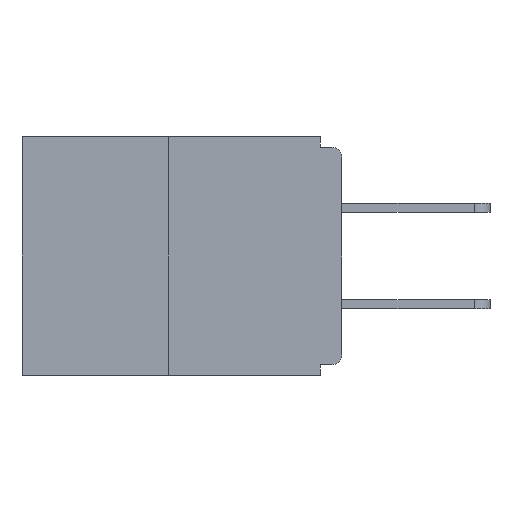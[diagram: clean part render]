
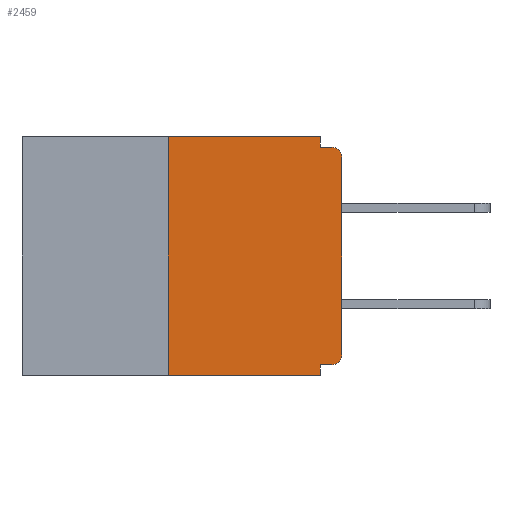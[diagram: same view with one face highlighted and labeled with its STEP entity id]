
A CAD part, left-side view. The second image highlights one B-rep face of the part: STEP entity #2459.
In plain terms, the highlighted planar face has unit normal (-1, 0, 0).
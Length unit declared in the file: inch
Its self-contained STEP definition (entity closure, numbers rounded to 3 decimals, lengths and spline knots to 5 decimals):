
#286 = DIRECTION ( 'NONE',  ( 0., 1., 0. ) ) ;
#424 = ORIENTED_EDGE ( 'NONE', *, *, #5537, .F. ) ;
#671 = CARTESIAN_POINT ( 'NONE',  ( 0., 0.015, -0.015 ) ) ;
#722 = FACE_OUTER_BOUND ( 'NONE', #28227, .T. ) ;
#727 = VECTOR ( 'NONE', #286, 39.37008 ) ;
#1129 = CARTESIAN_POINT ( 'NONE',  ( 0., 0., -0.015 ) ) ;
#1181 = ORIENTED_EDGE ( 'NONE', *, *, #14815, .F. ) ;
#1460 = EDGE_CURVE ( 'NONE', #25315, #20124, #7618, .T. ) ;
#1823 = VECTOR ( 'NONE', #16786, 39.37008 ) ;
#1989 = CARTESIAN_POINT ( 'NONE',  ( 0., 0.031, -0.343 ) ) ;
#2459 = ADVANCED_FACE ( 'NONE', ( #722 ), #16850, .F. ) ;
#2761 = VERTEX_POINT ( 'NONE', #17500 ) ;
#2852 = AXIS2_PLACEMENT_3D ( 'NONE', #22401, #15480, #24294 ) ;
#2941 = EDGE_CURVE ( 'NONE', #11455, #20124, #27939, .T. ) ;
#3742 = LINE ( 'NONE', #1129, #14697 ) ;
#5002 = VERTEX_POINT ( 'NONE', #21702 ) ;
#5537 = EDGE_CURVE ( 'NONE', #5002, #10292, #3742, .T. ) ;
#5964 = VECTOR ( 'NONE', #25538, 39.37008 ) ;
#6502 = LINE ( 'NONE', #23472, #727 ) ;
#7047 = VECTOR ( 'NONE', #24822, 39.37008 ) ;
#7618 = LINE ( 'NONE', #16416, #1823 ) ;
#8114 = VERTEX_POINT ( 'NONE', #12884 ) ;
#9465 = LINE ( 'NONE', #18548, #26489 ) ;
#9606 = VERTEX_POINT ( 'NONE', #20436 ) ;
#9784 = EDGE_CURVE ( 'NONE', #27364, #8114, #26362, .T. ) ;
#9930 = AXIS2_PLACEMENT_3D ( 'NONE', #20778, #27370, #12693 ) ;
#10292 = VERTEX_POINT ( 'NONE', #671 ) ;
#10309 = CARTESIAN_POINT ( 'NONE',  ( 0., 0.031, 0. ) ) ;
#10403 = LINE ( 'NONE', #10309, #5964 ) ;
#10485 = ORIENTED_EDGE ( 'NONE', *, *, #18618, .F. ) ;
#11455 = VERTEX_POINT ( 'NONE', #25111 ) ;
#11593 = VECTOR ( 'NONE', #18915, 39.37008 ) ;
#11884 = CARTESIAN_POINT ( 'NONE',  ( 0., 0.25, 0. ) ) ;
#12365 = CARTESIAN_POINT ( 'NONE',  ( 0., 0.46, 0. ) ) ;
#12693 = DIRECTION ( 'NONE',  ( 0., 0., -1. ) ) ;
#12884 = CARTESIAN_POINT ( 'NONE',  ( 0., 0., -0.313 ) ) ;
#14094 = VERTEX_POINT ( 'NONE', #11884 ) ;
#14412 = DIRECTION ( 'NONE',  ( 0., -1., 0. ) ) ;
#14697 = VECTOR ( 'NONE', #14412, 39.37008 ) ;
#14815 = EDGE_CURVE ( 'NONE', #9606, #5002, #10403, .T. ) ;
#15480 = DIRECTION ( 'NONE',  ( 1., 0., 0. ) ) ;
#15795 = DIRECTION ( 'NONE',  ( 0., 0., -1. ) ) ;
#16416 = CARTESIAN_POINT ( 'NONE',  ( 0., 0.031, -0.343 ) ) ;
#16460 = CARTESIAN_POINT ( 'NONE',  ( 0., 0.25, 0. ) ) ;
#16786 = DIRECTION ( 'NONE',  ( 0., 0., -1. ) ) ;
#16850 = PLANE ( 'NONE',  #2852 ) ;
#16987 = DIRECTION ( 'NONE',  ( 0., -1., 0. ) ) ;
#17480 = ORIENTED_EDGE ( 'NONE', *, *, #2941, .T. ) ;
#17500 = CARTESIAN_POINT ( 'NONE',  ( 0., 0., -0.03 ) ) ;
#17510 = ORIENTED_EDGE ( 'NONE', *, *, #9784, .T. ) ;
#18422 = ORIENTED_EDGE ( 'NONE', *, *, #21687, .F. ) ;
#18548 = CARTESIAN_POINT ( 'NONE',  ( 0., 0., 0. ) ) ;
#18618 = EDGE_CURVE ( 'NONE', #27364, #25315, #6502, .T. ) ;
#18915 = DIRECTION ( 'NONE',  ( 0., -1., 0. ) ) ;
#19212 = ORIENTED_EDGE ( 'NONE', *, *, #1460, .F. ) ;
#20124 = VERTEX_POINT ( 'NONE', #1989 ) ;
#20436 = CARTESIAN_POINT ( 'NONE',  ( 0., 0.031, 0. ) ) ;
#20461 = VECTOR ( 'NONE', #16987, 39.37008 ) ;
#20546 = DIRECTION ( 'NONE',  ( 0., 0., 1. ) ) ;
#20617 = EDGE_CURVE ( 'NONE', #14094, #9606, #23150, .T. ) ;
#20770 = ORIENTED_EDGE ( 'NONE', *, *, #20617, .F. ) ;
#20778 = CARTESIAN_POINT ( 'NONE',  ( 0., 0.015, -0.313 ) ) ;
#21568 = EDGE_CURVE ( 'NONE', #8114, #2761, #9465, .T. ) ;
#21687 = EDGE_CURVE ( 'NONE', #11455, #14094, #24433, .T. ) ;
#21702 = CARTESIAN_POINT ( 'NONE',  ( 0., 0.031, -0.015 ) ) ;
#22265 = CARTESIAN_POINT ( 'NONE',  ( 0., 0.015, -0.03 ) ) ;
#22401 = CARTESIAN_POINT ( 'NONE',  ( 0., 0.46, 0. ) ) ;
#23127 = EDGE_CURVE ( 'NONE', #2761, #10292, #24632, .T. ) ;
#23150 = LINE ( 'NONE', #12365, #11593 ) ;
#23319 = ORIENTED_EDGE ( 'NONE', *, *, #23127, .T. ) ;
#23472 = CARTESIAN_POINT ( 'NONE',  ( 0., 0., -0.328 ) ) ;
#23640 = CARTESIAN_POINT ( 'NONE',  ( 0., 0.46, -0.343 ) ) ;
#24294 = DIRECTION ( 'NONE',  ( 0., 0., -1. ) ) ;
#24433 = LINE ( 'NONE', #16460, #7047 ) ;
#24632 = CIRCLE ( 'NONE', #26239, 0.015 ) ;
#24742 = CARTESIAN_POINT ( 'NONE',  ( 0., 0.015, -0.328 ) ) ;
#24822 = DIRECTION ( 'NONE',  ( 0., 0., 1. ) ) ;
#25111 = CARTESIAN_POINT ( 'NONE',  ( 0., 0.25, -0.343 ) ) ;
#25315 = VERTEX_POINT ( 'NONE', #26916 ) ;
#25538 = DIRECTION ( 'NONE',  ( 0., 0., -1. ) ) ;
#26239 = AXIS2_PLACEMENT_3D ( 'NONE', #22265, #26931, #15795 ) ;
#26362 = CIRCLE ( 'NONE', #9930, 0.015 ) ;
#26489 = VECTOR ( 'NONE', #20546, 39.37008 ) ;
#26916 = CARTESIAN_POINT ( 'NONE',  ( 0., 0.031, -0.328 ) ) ;
#26931 = DIRECTION ( 'NONE',  ( -1., 0., 0. ) ) ;
#27364 = VERTEX_POINT ( 'NONE', #24742 ) ;
#27370 = DIRECTION ( 'NONE',  ( -1., 0., 0. ) ) ;
#27489 = ORIENTED_EDGE ( 'NONE', *, *, #21568, .T. ) ;
#27939 = LINE ( 'NONE', #23640, #20461 ) ;
#28227 = EDGE_LOOP ( 'NONE', ( #20770, #18422, #17480, #19212, #10485, #17510, #27489, #23319, #424, #1181 ) ) ;
